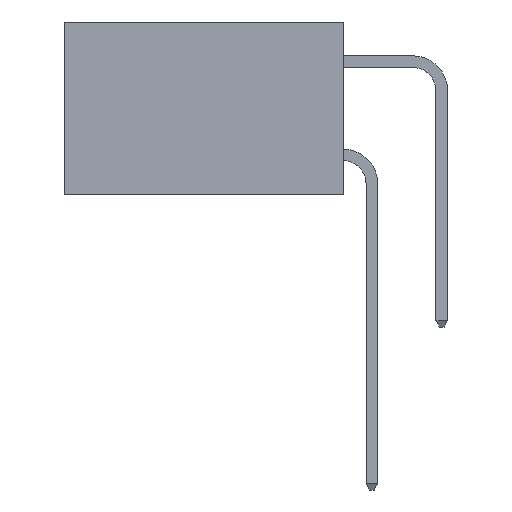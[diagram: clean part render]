
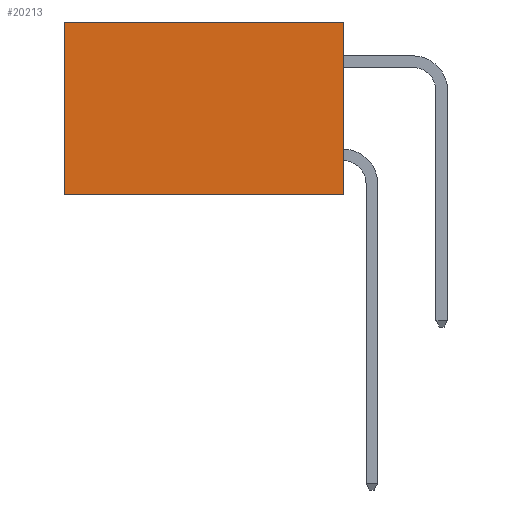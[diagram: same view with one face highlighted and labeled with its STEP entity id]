
A CAD part, left-side view. The second image highlights one B-rep face of the part: STEP entity #20213.
In plain terms, the highlighted planar face has unit normal (-1, 0, 0).
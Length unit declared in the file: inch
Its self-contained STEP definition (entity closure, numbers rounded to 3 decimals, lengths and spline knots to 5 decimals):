
#1009 = DIRECTION ( 'NONE',  ( 0., 1., 0. ) ) ;
#1053 = PLANE ( 'NONE',  #2336 ) ;
#1277 = ORIENTED_EDGE ( 'NONE', *, *, #7785, .F. ) ;
#2336 = AXIS2_PLACEMENT_3D ( 'NONE', #19727, #9839, #21335 ) ;
#2611 = EDGE_CURVE ( 'NONE', #20861, #9021, #9080, .T. ) ;
#4388 = EDGE_CURVE ( 'NONE', #20861, #12180, #10727, .T. ) ;
#4527 = VECTOR ( 'NONE', #18724, 39.37008 ) ;
#5254 = EDGE_LOOP ( 'NONE', ( #5512, #1277, #10891, #9321 ) ) ;
#5512 = ORIENTED_EDGE ( 'NONE', *, *, #5953, .T. ) ;
#5953 = EDGE_CURVE ( 'NONE', #12180, #21628, #8570, .T. ) ;
#6233 = VECTOR ( 'NONE', #16322, 39.37008 ) ;
#7702 = CARTESIAN_POINT ( 'NONE',  ( 0.2615, 0., -0.37 ) ) ;
#7785 = EDGE_CURVE ( 'NONE', #9021, #21628, #8764, .T. ) ;
#8046 = VECTOR ( 'NONE', #20420, 39.37008 ) ;
#8570 = LINE ( 'NONE', #20004, #8046 ) ;
#8764 = LINE ( 'NONE', #11406, #20884 ) ;
#9021 = VERTEX_POINT ( 'NONE', #7702 ) ;
#9080 = LINE ( 'NONE', #18341, #4527 ) ;
#9321 = ORIENTED_EDGE ( 'NONE', *, *, #4388, .T. ) ;
#9839 = DIRECTION ( 'NONE',  ( 1., 0., 0. ) ) ;
#10328 = CARTESIAN_POINT ( 'NONE',  ( 0.2615, 0.6, 0. ) ) ;
#10727 = LINE ( 'NONE', #16055, #6233 ) ;
#10891 = ORIENTED_EDGE ( 'NONE', *, *, #2611, .F. ) ;
#11406 = CARTESIAN_POINT ( 'NONE',  ( 0.2615, 0., -0.37 ) ) ;
#12180 = VERTEX_POINT ( 'NONE', #10328 ) ;
#14819 = CARTESIAN_POINT ( 'NONE',  ( 0.2615, 0., 0. ) ) ;
#15121 = FACE_OUTER_BOUND ( 'NONE', #5254, .T. ) ;
#16055 = CARTESIAN_POINT ( 'NONE',  ( 0.2615, 0., 0. ) ) ;
#16322 = DIRECTION ( 'NONE',  ( 0., 1., 0. ) ) ;
#18341 = CARTESIAN_POINT ( 'NONE',  ( 0.2615, 0., -0.37 ) ) ;
#18724 = DIRECTION ( 'NONE',  ( 0., 0., -1. ) ) ;
#19727 = CARTESIAN_POINT ( 'NONE',  ( 0.2615, 0., -0.37 ) ) ;
#20004 = CARTESIAN_POINT ( 'NONE',  ( 0.2615, 0.6, -0.37 ) ) ;
#20213 = ADVANCED_FACE ( 'NONE', ( #15121 ), #1053, .F. ) ;
#20420 = DIRECTION ( 'NONE',  ( 0., 0., -1. ) ) ;
#20861 = VERTEX_POINT ( 'NONE', #14819 ) ;
#20884 = VECTOR ( 'NONE', #1009, 39.37008 ) ;
#21335 = DIRECTION ( 'NONE',  ( 0., 0., -1. ) ) ;
#21426 = CARTESIAN_POINT ( 'NONE',  ( 0.2615, 0.6, -0.37 ) ) ;
#21628 = VERTEX_POINT ( 'NONE', #21426 ) ;
